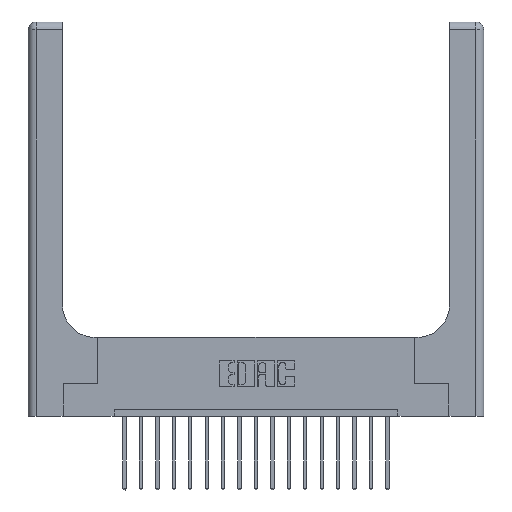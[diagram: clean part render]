
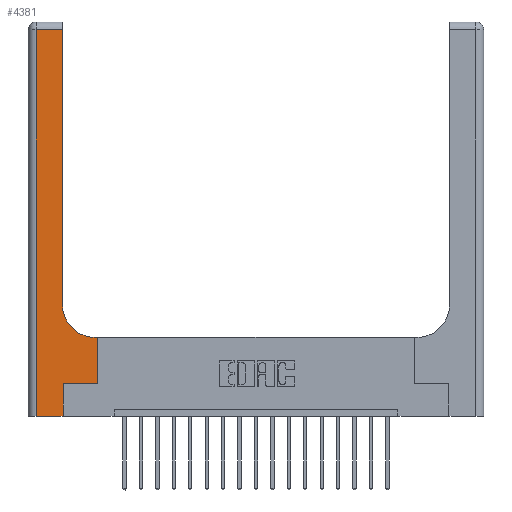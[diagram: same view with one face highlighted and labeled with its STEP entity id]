
A CAD part, top view. The second image highlights one B-rep face of the part: STEP entity #4381.
In plain terms, the highlighted planar face has unit normal (0, 0, 1).
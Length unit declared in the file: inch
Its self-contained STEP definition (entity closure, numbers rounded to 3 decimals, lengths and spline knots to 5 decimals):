
#51 = CARTESIAN_POINT ( 'NONE',  ( 0.26, 0.6, 0.37 ) ) ;
#86 = CARTESIAN_POINT ( 'NONE',  ( 0., 3., 0.37 ) ) ;
#282 = CARTESIAN_POINT ( 'NONE',  ( 0.265, 0.25, 0.37 ) ) ;
#520 = VECTOR ( 'NONE', #10219, 39.37008 ) ;
#870 = VECTOR ( 'NONE', #5040, 39.37008 ) ;
#1334 = ORIENTED_EDGE ( 'NONE', *, *, #17650, .T. ) ;
#1550 = CARTESIAN_POINT ( 'NONE',  ( 0.528, 0.6, 0.37 ) ) ;
#1575 = VECTOR ( 'NONE', #7876, 39.37008 ) ;
#1746 = CARTESIAN_POINT ( 'NONE',  ( 0.26, 0.85, 0.37 ) ) ;
#1925 = CARTESIAN_POINT ( 'NONE',  ( 0.51, 0.85, 0.37 ) ) ;
#1990 = VECTOR ( 'NONE', #2871, 39.37008 ) ;
#2153 = EDGE_LOOP ( 'NONE', ( #1334, #6262, #17127, #10317, #4945, #12968, #17531, #15628, #4317 ) ) ;
#2252 = EDGE_CURVE ( 'NONE', #14135, #2959, #9867, .T. ) ;
#2739 = AXIS2_PLACEMENT_3D ( 'NONE', #86, #14774, #11966 ) ;
#2871 = DIRECTION ( 'NONE',  ( -1., 0., 0. ) ) ;
#2959 = VERTEX_POINT ( 'NONE', #12153 ) ;
#4180 = VECTOR ( 'NONE', #5481, 39.37008 ) ;
#4317 = ORIENTED_EDGE ( 'NONE', *, *, #16081, .T. ) ;
#4381 = ADVANCED_FACE ( 'NONE', ( #17265 ), #10316, .F. ) ;
#4386 = VERTEX_POINT ( 'NONE', #1550 ) ;
#4945 = ORIENTED_EDGE ( 'NONE', *, *, #2252, .T. ) ;
#5040 = DIRECTION ( 'NONE',  ( -1., 0., 0. ) ) ;
#5481 = DIRECTION ( 'NONE',  ( 0., -1., 0. ) ) ;
#5912 = LINE ( 'NONE', #6444, #870 ) ;
#6262 = ORIENTED_EDGE ( 'NONE', *, *, #14010, .T. ) ;
#6444 = CARTESIAN_POINT ( 'NONE',  ( 0., 2.94, 0.37 ) ) ;
#6571 = LINE ( 'NONE', #282, #17688 ) ;
#6630 = EDGE_CURVE ( 'NONE', #9494, #4386, #14591, .T. ) ;
#7084 = CARTESIAN_POINT ( 'NONE',  ( 0.265, 0., 0.37 ) ) ;
#7876 = DIRECTION ( 'NONE',  ( 0., 1., 0. ) ) ;
#7903 = VECTOR ( 'NONE', #15342, 39.37008 ) ;
#7959 = CIRCLE ( 'NONE', #16987, 0.25 ) ;
#8498 = CARTESIAN_POINT ( 'NONE',  ( 0.26, 3., 0.37 ) ) ;
#8791 = VECTOR ( 'NONE', #10101, 39.37008 ) ;
#9491 = VERTEX_POINT ( 'NONE', #18422 ) ;
#9494 = VERTEX_POINT ( 'NONE', #15614 ) ;
#9626 = VERTEX_POINT ( 'NONE', #16070 ) ;
#9692 = EDGE_CURVE ( 'NONE', #9626, #14135, #10644, .T. ) ;
#9836 = DIRECTION ( 'NONE',  ( 1., 0., 0. ) ) ;
#9867 = LINE ( 'NONE', #18074, #1575 ) ;
#10101 = DIRECTION ( 'NONE',  ( 1., 0., 0. ) ) ;
#10219 = DIRECTION ( 'NONE',  ( 0., 1., 0. ) ) ;
#10316 = PLANE ( 'NONE',  #2739 ) ;
#10317 = ORIENTED_EDGE ( 'NONE', *, *, #9692, .T. ) ;
#10644 = LINE ( 'NONE', #11610, #8791 ) ;
#11313 = CARTESIAN_POINT ( 'NONE',  ( 0.06, 3., 0.37 ) ) ;
#11610 = CARTESIAN_POINT ( 'NONE',  ( 0., 0., 0.37 ) ) ;
#11966 = DIRECTION ( 'NONE',  ( -1., 0., 0. ) ) ;
#12153 = CARTESIAN_POINT ( 'NONE',  ( 0.265, 0.25, 0.37 ) ) ;
#12525 = LINE ( 'NONE', #11313, #4180 ) ;
#12765 = EDGE_CURVE ( 'NONE', #4386, #9491, #15393, .T. ) ;
#12968 = ORIENTED_EDGE ( 'NONE', *, *, #15923, .T. ) ;
#13072 = CARTESIAN_POINT ( 'NONE',  ( 0.26, 2.94, 0.37 ) ) ;
#13179 = LINE ( 'NONE', #8498, #520 ) ;
#14010 = EDGE_CURVE ( 'NONE', #14434, #17478, #5912, .T. ) ;
#14109 = CARTESIAN_POINT ( 'NONE',  ( 0.06, 2.94, 0.37 ) ) ;
#14135 = VERTEX_POINT ( 'NONE', #7084 ) ;
#14434 = VERTEX_POINT ( 'NONE', #13072 ) ;
#14591 = LINE ( 'NONE', #15280, #7903 ) ;
#14774 = DIRECTION ( 'NONE',  ( 0., 0., -1. ) ) ;
#15280 = CARTESIAN_POINT ( 'NONE',  ( 0.528, 0.25, 0.37 ) ) ;
#15342 = DIRECTION ( 'NONE',  ( 0., 1., 0. ) ) ;
#15393 = LINE ( 'NONE', #51, #1990 ) ;
#15614 = CARTESIAN_POINT ( 'NONE',  ( 0.528, 0.25, 0.37 ) ) ;
#15628 = ORIENTED_EDGE ( 'NONE', *, *, #12765, .T. ) ;
#15923 = EDGE_CURVE ( 'NONE', #2959, #9494, #6571, .T. ) ;
#16070 = CARTESIAN_POINT ( 'NONE',  ( 0.06, 0., 0.37 ) ) ;
#16081 = EDGE_CURVE ( 'NONE', #9491, #16297, #7959, .T. ) ;
#16297 = VERTEX_POINT ( 'NONE', #1746 ) ;
#16987 = AXIS2_PLACEMENT_3D ( 'NONE', #1925, #17059, #9836 ) ;
#17059 = DIRECTION ( 'NONE',  ( 0., 0., -1. ) ) ;
#17127 = ORIENTED_EDGE ( 'NONE', *, *, #17952, .T. ) ;
#17265 = FACE_OUTER_BOUND ( 'NONE', #2153, .T. ) ;
#17478 = VERTEX_POINT ( 'NONE', #14109 ) ;
#17531 = ORIENTED_EDGE ( 'NONE', *, *, #6630, .T. ) ;
#17650 = EDGE_CURVE ( 'NONE', #16297, #14434, #13179, .T. ) ;
#17688 = VECTOR ( 'NONE', #18147, 39.37008 ) ;
#17952 = EDGE_CURVE ( 'NONE', #17478, #9626, #12525, .T. ) ;
#18074 = CARTESIAN_POINT ( 'NONE',  ( 0.265, 0., 0.37 ) ) ;
#18147 = DIRECTION ( 'NONE',  ( 1., 0., 0. ) ) ;
#18422 = CARTESIAN_POINT ( 'NONE',  ( 0.51, 0.6, 0.37 ) ) ;
